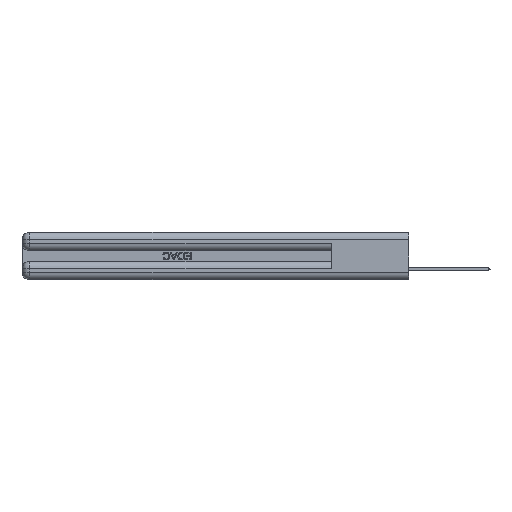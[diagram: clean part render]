
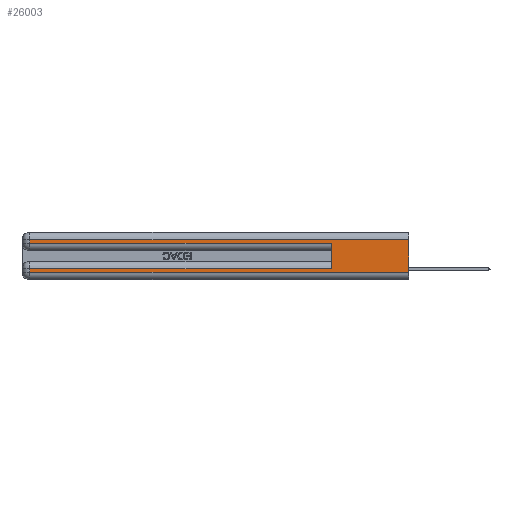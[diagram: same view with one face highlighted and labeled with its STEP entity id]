
A CAD part, left-side view. The second image highlights one B-rep face of the part: STEP entity #26003.
In plain terms, the highlighted planar face has unit normal (-1, 0, 0).
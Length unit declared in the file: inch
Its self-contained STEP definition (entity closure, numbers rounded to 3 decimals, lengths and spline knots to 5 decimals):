
#1872 = VERTEX_POINT ( 'NONE', #29100 ) ;
#1981 = LINE ( 'NONE', #37975, #7167 ) ;
#3770 = DIRECTION ( 'NONE',  ( 1., 0., 0. ) ) ;
#5106 = ORIENTED_EDGE ( 'NONE', *, *, #47063, .T. ) ;
#5682 = VERTEX_POINT ( 'NONE', #9584 ) ;
#7167 = VECTOR ( 'NONE', #50721, 39.37008 ) ;
#7650 = LINE ( 'NONE', #12985, #13413 ) ;
#7724 = PLANE ( 'NONE',  #9287 ) ;
#7886 = VERTEX_POINT ( 'NONE', #13726 ) ;
#7908 = DIRECTION ( 'NONE',  ( 0., 0., -1. ) ) ;
#8184 = CARTESIAN_POINT ( 'NONE',  ( 0., 2.94, 0.37 ) ) ;
#9262 = EDGE_CURVE ( 'NONE', #24590, #45942, #26628, .T. ) ;
#9287 = AXIS2_PLACEMENT_3D ( 'NONE', #19602, #3770, #7908 ) ;
#9584 = CARTESIAN_POINT ( 'NONE',  ( 0., 0., 0.06 ) ) ;
#9988 = CARTESIAN_POINT ( 'NONE',  ( 0., 2.94, 0.285 ) ) ;
#11300 = VERTEX_POINT ( 'NONE', #33952 ) ;
#11511 = EDGE_CURVE ( 'NONE', #39365, #24590, #7650, .T. ) ;
#11735 = VERTEX_POINT ( 'NONE', #27866 ) ;
#12316 = DIRECTION ( 'NONE',  ( 0., 0., 1. ) ) ;
#12926 = DIRECTION ( 'NONE',  ( 0., -1., 0. ) ) ;
#12985 = CARTESIAN_POINT ( 'NONE',  ( 0., 2.94, 0.37 ) ) ;
#13328 = EDGE_LOOP ( 'NONE', ( #52578, #47536, #34426, #26917, #27829, #5106, #15201, #53359 ) ) ;
#13337 = DIRECTION ( 'NONE',  ( 0., 0., -1. ) ) ;
#13413 = VECTOR ( 'NONE', #13337, 39.37008 ) ;
#13726 = CARTESIAN_POINT ( 'NONE',  ( 0., 0.6, 0.085 ) ) ;
#14684 = DIRECTION ( 'NONE',  ( 0., 1., 0. ) ) ;
#15201 = ORIENTED_EDGE ( 'NONE', *, *, #30547, .T. ) ;
#15615 = EDGE_CURVE ( 'NONE', #11300, #5682, #1981, .T. ) ;
#17656 = LINE ( 'NONE', #49610, #19632 ) ;
#18210 = VECTOR ( 'NONE', #38480, 39.37008 ) ;
#19602 = CARTESIAN_POINT ( 'NONE',  ( 0., 0., 0.37 ) ) ;
#19632 = VECTOR ( 'NONE', #12926, 39.37008 ) ;
#19749 = LINE ( 'NONE', #27161, #41139 ) ;
#20090 = LINE ( 'NONE', #8184, #42650 ) ;
#21754 = LINE ( 'NONE', #36896, #47618 ) ;
#23352 = CARTESIAN_POINT ( 'NONE',  ( 0., 0., 0.085 ) ) ;
#24590 = VERTEX_POINT ( 'NONE', #9988 ) ;
#26003 = ADVANCED_FACE ( 'NONE', ( #52204 ), #7724, .F. ) ;
#26239 = CARTESIAN_POINT ( 'NONE',  ( 0., 0.6, 0.285 ) ) ;
#26628 = LINE ( 'NONE', #42945, #18210 ) ;
#26917 = ORIENTED_EDGE ( 'NONE', *, *, #9262, .T. ) ;
#27161 = CARTESIAN_POINT ( 'NONE',  ( 0., 0., 0.31 ) ) ;
#27829 = ORIENTED_EDGE ( 'NONE', *, *, #51070, .F. ) ;
#27866 = CARTESIAN_POINT ( 'NONE',  ( 0., 2.94, 0.085 ) ) ;
#28998 = CARTESIAN_POINT ( 'NONE',  ( 0., 2.94, 0.31 ) ) ;
#29100 = CARTESIAN_POINT ( 'NONE',  ( 0., 2.94, 0.06 ) ) ;
#30547 = EDGE_CURVE ( 'NONE', #11735, #1872, #20090, .T. ) ;
#33952 = CARTESIAN_POINT ( 'NONE',  ( 0., 0., 0.31 ) ) ;
#34426 = ORIENTED_EDGE ( 'NONE', *, *, #11511, .T. ) ;
#34433 = LINE ( 'NONE', #23352, #44149 ) ;
#35808 = DIRECTION ( 'NONE',  ( 0., 1., 0. ) ) ;
#35949 = EDGE_CURVE ( 'NONE', #1872, #5682, #17656, .T. ) ;
#36896 = CARTESIAN_POINT ( 'NONE',  ( 0., 0.6, 0.145 ) ) ;
#37975 = CARTESIAN_POINT ( 'NONE',  ( 0., 0., 0.37 ) ) ;
#38480 = DIRECTION ( 'NONE',  ( 0., -1., 0. ) ) ;
#39365 = VERTEX_POINT ( 'NONE', #28998 ) ;
#41139 = VECTOR ( 'NONE', #14684, 39.37008 ) ;
#42650 = VECTOR ( 'NONE', #44491, 39.37008 ) ;
#42945 = CARTESIAN_POINT ( 'NONE',  ( 0., 0., 0.285 ) ) ;
#44149 = VECTOR ( 'NONE', #35808, 39.37008 ) ;
#44491 = DIRECTION ( 'NONE',  ( 0., 0., -1. ) ) ;
#45942 = VERTEX_POINT ( 'NONE', #26239 ) ;
#47063 = EDGE_CURVE ( 'NONE', #7886, #11735, #34433, .T. ) ;
#47536 = ORIENTED_EDGE ( 'NONE', *, *, #51741, .T. ) ;
#47618 = VECTOR ( 'NONE', #12316, 39.37008 ) ;
#49610 = CARTESIAN_POINT ( 'NONE',  ( 0., 0., 0.06 ) ) ;
#50721 = DIRECTION ( 'NONE',  ( 0., 0., -1. ) ) ;
#51070 = EDGE_CURVE ( 'NONE', #7886, #45942, #21754, .T. ) ;
#51741 = EDGE_CURVE ( 'NONE', #11300, #39365, #19749, .T. ) ;
#52204 = FACE_OUTER_BOUND ( 'NONE', #13328, .T. ) ;
#52578 = ORIENTED_EDGE ( 'NONE', *, *, #15615, .F. ) ;
#53359 = ORIENTED_EDGE ( 'NONE', *, *, #35949, .T. ) ;
